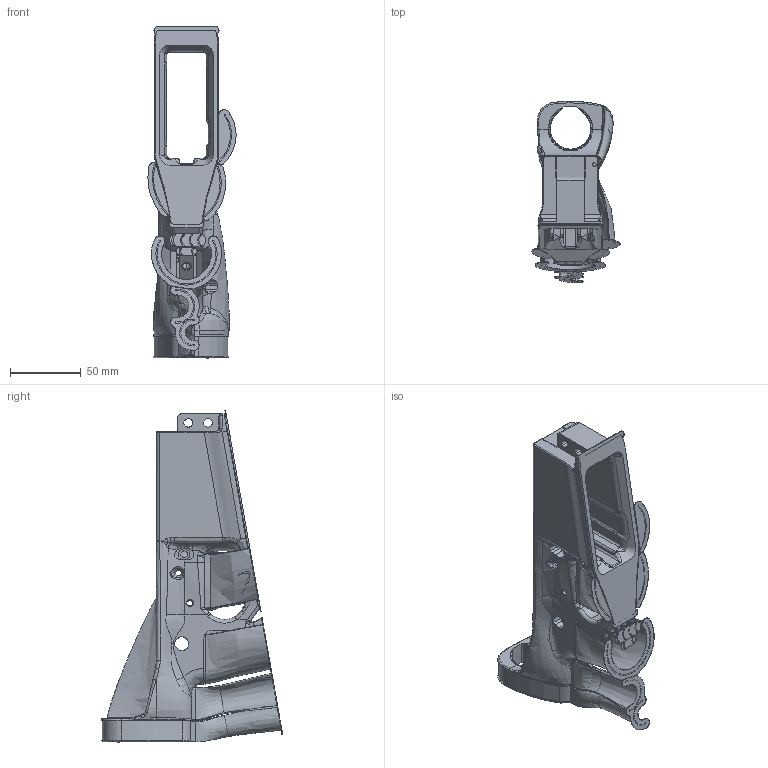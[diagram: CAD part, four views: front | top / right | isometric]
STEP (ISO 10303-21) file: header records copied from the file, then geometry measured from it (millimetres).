
FILE_DESCRIPTION (( 'STEP AP203' ), '1' );
FILE_NAME ('LR-308 BL V2.6.STEP', '2022-05-15T13:42:22', ( '' ), ( '' ), 'SwSTEP 2.0', 'SolidWorks 2021', '' );
FILE_SCHEMA (( 'CONFIG_CONTROL_DESIGN' ));
Products named in the file (1): LR-308 BL V2.6
Bounding box: 62.42 x 128.11 x 234.71 mm (x, y, z)
Volume: 220570.5 mm3; surface area: 112997.5 mm2
Topology: 8 solids, 8 shells, 2106 faces, 5764 edges, 3699 vertices
Faces by surface type: bspline 1025, plane 617, cylinder 373, torus 53, cone 28, sphere 10
Entity records: 229980 total; most frequent: CARTESIAN_POINT 185239, ORIENTED_EDGE 11410, DIRECTION 5975, EDGE_CURVE 5705, VERTEX_POINT 3699, B_SPLINE_CURVE_WITH_KNOTS 2460, VECTOR 2243, LINE 2243
